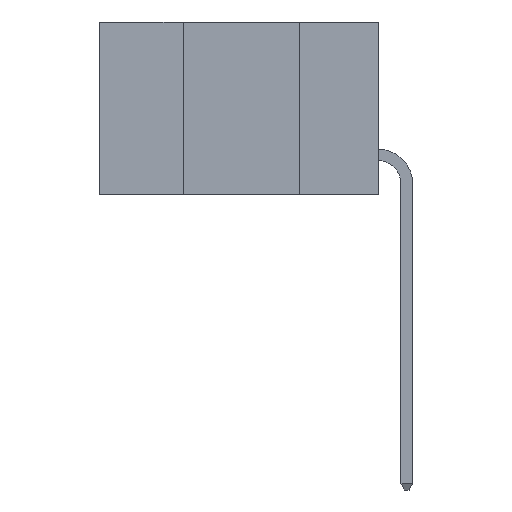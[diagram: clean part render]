
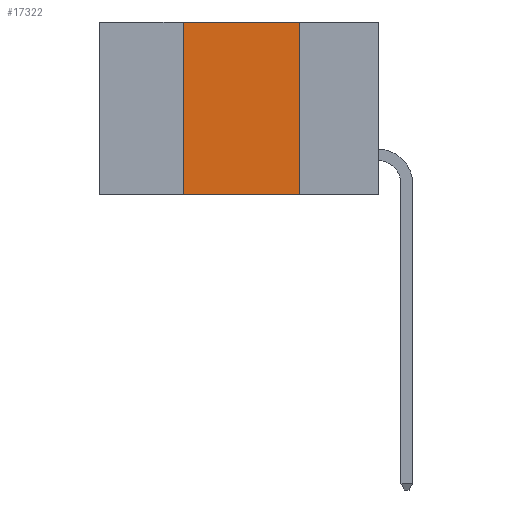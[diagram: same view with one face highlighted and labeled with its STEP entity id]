
A CAD part, left-side view. The second image highlights one B-rep face of the part: STEP entity #17322.
In plain terms, the highlighted planar face has unit normal (-1, 0, 0).
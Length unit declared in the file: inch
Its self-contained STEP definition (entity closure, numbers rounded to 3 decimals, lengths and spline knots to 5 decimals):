
#477 = LINE ( 'NONE', #15542, #4117 ) ;
#754 = VERTEX_POINT ( 'NONE', #10936 ) ;
#963 = EDGE_CURVE ( 'NONE', #17054, #17481, #18328, .T. ) ;
#1010 = CARTESIAN_POINT ( 'NONE',  ( 0., 0.6, 0. ) ) ;
#2568 = DIRECTION ( 'NONE',  ( 0., 0., 1. ) ) ;
#2569 = DIRECTION ( 'NONE',  ( 1., 0., 0. ) ) ;
#2686 = LINE ( 'NONE', #18586, #3174 ) ;
#2853 = ORIENTED_EDGE ( 'NONE', *, *, #12907, .F. ) ;
#3174 = VECTOR ( 'NONE', #11222, 39.37008 ) ;
#4117 = VECTOR ( 'NONE', #8126, 39.37008 ) ;
#4162 = VERTEX_POINT ( 'NONE', #16969 ) ;
#5067 = ORIENTED_EDGE ( 'NONE', *, *, #19134, .F. ) ;
#7184 = ORIENTED_EDGE ( 'NONE', *, *, #18227, .T. ) ;
#7612 = DIRECTION ( 'NONE',  ( 0., -1., 0. ) ) ;
#7744 = LINE ( 'NONE', #13553, #15201 ) ;
#7765 = ORIENTED_EDGE ( 'NONE', *, *, #963, .F. ) ;
#8126 = DIRECTION ( 'NONE',  ( 0., -1., 0. ) ) ;
#10516 = CARTESIAN_POINT ( 'NONE',  ( 0., 0.42, 0. ) ) ;
#10936 = CARTESIAN_POINT ( 'NONE',  ( 0., 0.17, -0.37 ) ) ;
#10997 = FACE_OUTER_BOUND ( 'NONE', #14992, .T. ) ;
#11222 = DIRECTION ( 'NONE',  ( 0., 0., -1. ) ) ;
#12907 = EDGE_CURVE ( 'NONE', #17481, #4162, #477, .T. ) ;
#13127 = DIRECTION ( 'NONE',  ( 0., 0., -1. ) ) ;
#13553 = CARTESIAN_POINT ( 'NONE',  ( 0., 0.6, -0.37 ) ) ;
#14433 = CARTESIAN_POINT ( 'NONE',  ( 0., 0.42, -0.37 ) ) ;
#14566 = PLANE ( 'NONE',  #16655 ) ;
#14992 = EDGE_LOOP ( 'NONE', ( #5067, #2853, #7765, #7184 ) ) ;
#15201 = VECTOR ( 'NONE', #7612, 39.37008 ) ;
#15542 = CARTESIAN_POINT ( 'NONE',  ( 0., 0.6, 0. ) ) ;
#16655 = AXIS2_PLACEMENT_3D ( 'NONE', #1010, #2569, #13127 ) ;
#16862 = CARTESIAN_POINT ( 'NONE',  ( 0., 0.42, -0.37 ) ) ;
#16969 = CARTESIAN_POINT ( 'NONE',  ( 0., 0.17, 0. ) ) ;
#17054 = VERTEX_POINT ( 'NONE', #16862 ) ;
#17322 = ADVANCED_FACE ( 'NONE', ( #10997 ), #14566, .F. ) ;
#17481 = VERTEX_POINT ( 'NONE', #10516 ) ;
#17870 = VECTOR ( 'NONE', #2568, 39.37008 ) ;
#18227 = EDGE_CURVE ( 'NONE', #17054, #754, #7744, .T. ) ;
#18328 = LINE ( 'NONE', #14433, #17870 ) ;
#18586 = CARTESIAN_POINT ( 'NONE',  ( 0., 0.17, -0.37 ) ) ;
#19134 = EDGE_CURVE ( 'NONE', #4162, #754, #2686, .T. ) ;
